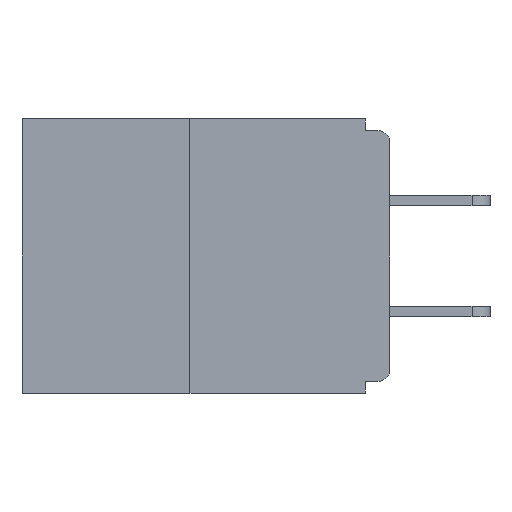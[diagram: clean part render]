
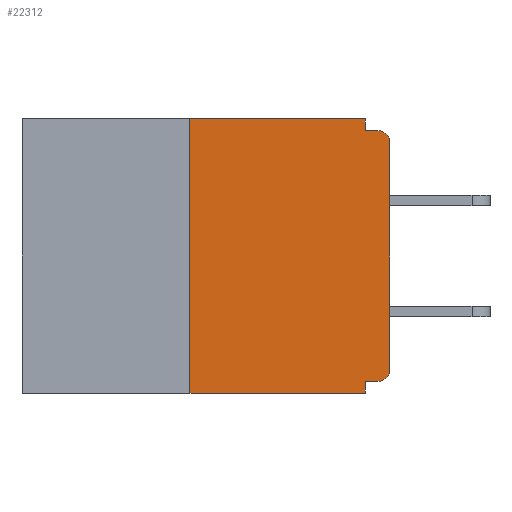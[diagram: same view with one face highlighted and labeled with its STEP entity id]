
A CAD part, left-side view. The second image highlights one B-rep face of the part: STEP entity #22312.
In plain terms, the highlighted planar face has unit normal (-1, 0, 0).
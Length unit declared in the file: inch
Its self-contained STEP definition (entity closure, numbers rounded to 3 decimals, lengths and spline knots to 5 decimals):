
#53 = EDGE_CURVE ( 'NONE', #8333, #16299, #20791, .T. ) ;
#187 = ORIENTED_EDGE ( 'NONE', *, *, #53, .T. ) ;
#312 = EDGE_CURVE ( 'NONE', #12813, #14544, #13982, .T. ) ;
#379 = DIRECTION ( 'NONE',  ( -1., 0., 0. ) ) ;
#745 = CARTESIAN_POINT ( 'NONE',  ( 0., 0., -0.03 ) ) ;
#1025 = CIRCLE ( 'NONE', #6629, 0.015 ) ;
#1902 = CARTESIAN_POINT ( 'NONE',  ( 0., 0., -0.015 ) ) ;
#2395 = AXIS2_PLACEMENT_3D ( 'NONE', #8314, #15955, #21405 ) ;
#2618 = CIRCLE ( 'NONE', #16292, 0.015 ) ;
#3435 = DIRECTION ( 'NONE',  ( 0., -1., 0. ) ) ;
#3584 = VERTEX_POINT ( 'NONE', #5823 ) ;
#3979 = LINE ( 'NONE', #9344, #11079 ) ;
#4204 = ORIENTED_EDGE ( 'NONE', *, *, #15410, .T. ) ;
#4780 = EDGE_CURVE ( 'NONE', #17537, #15793, #19452, .T. ) ;
#5034 = EDGE_CURVE ( 'NONE', #14544, #3584, #18306, .T. ) ;
#5158 = CARTESIAN_POINT ( 'NONE',  ( 0., 0., -0.313 ) ) ;
#5222 = VERTEX_POINT ( 'NONE', #18924 ) ;
#5822 = CARTESIAN_POINT ( 'NONE',  ( 0., 0.25, -0.343 ) ) ;
#5823 = CARTESIAN_POINT ( 'NONE',  ( 0., 0.015, -0.015 ) ) ;
#6022 = CARTESIAN_POINT ( 'NONE',  ( 0., 0.031, -0.343 ) ) ;
#6402 = VECTOR ( 'NONE', #22624, 39.37008 ) ;
#6435 = LINE ( 'NONE', #7804, #6997 ) ;
#6629 = AXIS2_PLACEMENT_3D ( 'NONE', #17635, #15964, #15883 ) ;
#6997 = VECTOR ( 'NONE', #13136, 39.37008 ) ;
#7092 = ORIENTED_EDGE ( 'NONE', *, *, #4780, .T. ) ;
#7804 = CARTESIAN_POINT ( 'NONE',  ( 0., 0.031, -0.343 ) ) ;
#8314 = CARTESIAN_POINT ( 'NONE',  ( 0., 0.46, 0. ) ) ;
#8333 = VERTEX_POINT ( 'NONE', #5822 ) ;
#8465 = CARTESIAN_POINT ( 'NONE',  ( 0., 0., 0. ) ) ;
#9283 = EDGE_CURVE ( 'NONE', #21216, #12813, #16035, .T. ) ;
#9344 = CARTESIAN_POINT ( 'NONE',  ( 0., 0.25, 0. ) ) ;
#9502 = CARTESIAN_POINT ( 'NONE',  ( 0., 0., -0.328 ) ) ;
#9717 = CARTESIAN_POINT ( 'NONE',  ( 0., 0.46, 0. ) ) ;
#9878 = CARTESIAN_POINT ( 'NONE',  ( 0., 0.031, -0.015 ) ) ;
#10173 = EDGE_LOOP ( 'NONE', ( #12305, #11954, #187, #22204, #14421, #4204, #7092, #10254, #21764, #17036 ) ) ;
#10254 = ORIENTED_EDGE ( 'NONE', *, *, #10823, .T. ) ;
#10292 = VECTOR ( 'NONE', #16547, 39.37008 ) ;
#10792 = LINE ( 'NONE', #9502, #15349 ) ;
#10823 = EDGE_CURVE ( 'NONE', #15793, #3584, #2618, .T. ) ;
#11079 = VECTOR ( 'NONE', #12919, 39.37008 ) ;
#11181 = VERTEX_POINT ( 'NONE', #16301 ) ;
#11328 = DIRECTION ( 'NONE',  ( 0., 1., 0. ) ) ;
#11462 = CARTESIAN_POINT ( 'NONE',  ( 0., 0.015, -0.03 ) ) ;
#11569 = CARTESIAN_POINT ( 'NONE',  ( 0., 0.46, -0.343 ) ) ;
#11842 = CARTESIAN_POINT ( 'NONE',  ( 0., 0.031, 0. ) ) ;
#11881 = EDGE_CURVE ( 'NONE', #11181, #5222, #10792, .T. ) ;
#11954 = ORIENTED_EDGE ( 'NONE', *, *, #22513, .F. ) ;
#12305 = ORIENTED_EDGE ( 'NONE', *, *, #9283, .F. ) ;
#12462 = PLANE ( 'NONE',  #2395 ) ;
#12813 = VERTEX_POINT ( 'NONE', #11842 ) ;
#12919 = DIRECTION ( 'NONE',  ( 0., 0., 1. ) ) ;
#13136 = DIRECTION ( 'NONE',  ( 0., 0., -1. ) ) ;
#13441 = VECTOR ( 'NONE', #3435, 39.37008 ) ;
#13982 = LINE ( 'NONE', #14724, #10292 ) ;
#14277 = EDGE_CURVE ( 'NONE', #5222, #16299, #6435, .T. ) ;
#14421 = ORIENTED_EDGE ( 'NONE', *, *, #11881, .F. ) ;
#14544 = VERTEX_POINT ( 'NONE', #9878 ) ;
#14724 = CARTESIAN_POINT ( 'NONE',  ( 0., 0.031, 0. ) ) ;
#15349 = VECTOR ( 'NONE', #11328, 39.37008 ) ;
#15410 = EDGE_CURVE ( 'NONE', #11181, #17537, #1025, .T. ) ;
#15793 = VERTEX_POINT ( 'NONE', #745 ) ;
#15883 = DIRECTION ( 'NONE',  ( 0., 0., -1. ) ) ;
#15955 = DIRECTION ( 'NONE',  ( 1., 0., 0. ) ) ;
#15964 = DIRECTION ( 'NONE',  ( -1., 0., 0. ) ) ;
#16035 = LINE ( 'NONE', #9717, #6402 ) ;
#16292 = AXIS2_PLACEMENT_3D ( 'NONE', #11462, #379, #22304 ) ;
#16299 = VERTEX_POINT ( 'NONE', #6022 ) ;
#16301 = CARTESIAN_POINT ( 'NONE',  ( 0., 0.015, -0.328 ) ) ;
#16490 = DIRECTION ( 'NONE',  ( 0., -1., 0. ) ) ;
#16547 = DIRECTION ( 'NONE',  ( 0., 0., -1. ) ) ;
#17036 = ORIENTED_EDGE ( 'NONE', *, *, #312, .F. ) ;
#17148 = CARTESIAN_POINT ( 'NONE',  ( 0., 0.25, 0. ) ) ;
#17453 = DIRECTION ( 'NONE',  ( 0., 0., 1. ) ) ;
#17537 = VERTEX_POINT ( 'NONE', #5158 ) ;
#17635 = CARTESIAN_POINT ( 'NONE',  ( 0., 0.015, -0.313 ) ) ;
#18306 = LINE ( 'NONE', #1902, #22244 ) ;
#18924 = CARTESIAN_POINT ( 'NONE',  ( 0., 0.031, -0.328 ) ) ;
#19452 = LINE ( 'NONE', #8465, #20581 ) ;
#20581 = VECTOR ( 'NONE', #17453, 39.37008 ) ;
#20752 = FACE_OUTER_BOUND ( 'NONE', #10173, .T. ) ;
#20791 = LINE ( 'NONE', #11569, #13441 ) ;
#21216 = VERTEX_POINT ( 'NONE', #17148 ) ;
#21405 = DIRECTION ( 'NONE',  ( 0., 0., -1. ) ) ;
#21764 = ORIENTED_EDGE ( 'NONE', *, *, #5034, .F. ) ;
#22204 = ORIENTED_EDGE ( 'NONE', *, *, #14277, .F. ) ;
#22244 = VECTOR ( 'NONE', #16490, 39.37008 ) ;
#22304 = DIRECTION ( 'NONE',  ( 0., 0., -1. ) ) ;
#22312 = ADVANCED_FACE ( 'NONE', ( #20752 ), #12462, .F. ) ;
#22513 = EDGE_CURVE ( 'NONE', #8333, #21216, #3979, .T. ) ;
#22624 = DIRECTION ( 'NONE',  ( 0., -1., 0. ) ) ;
